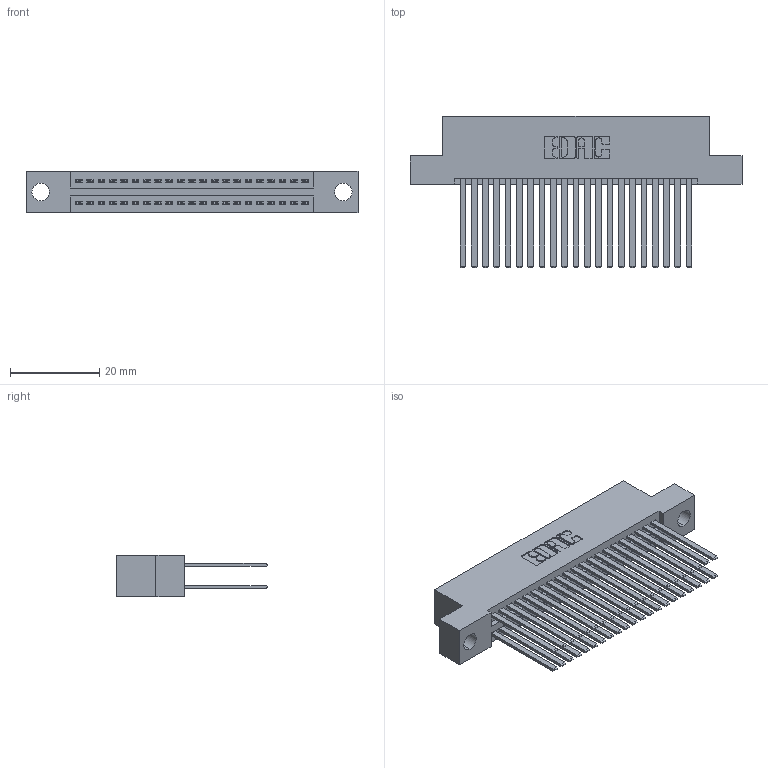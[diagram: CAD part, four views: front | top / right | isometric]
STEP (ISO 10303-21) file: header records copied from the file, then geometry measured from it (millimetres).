
FILE_DESCRIPTION (( 'STEP AP203' ), '1' );
FILE_NAME ('395-042-544-204.STEP', '2018-11-15T11:26:29', ( '' ), ( '' ), 'SwSTEP 2.0', 'SolidWorks 2016', '' );
FILE_SCHEMA (( 'CONFIG_CONTROL_DESIGN' ));
Length unit declared in the file: inch
Products named in the file (3): 345-292-001_345-293-144; 395-042-544-204; 345 Part_Flush Mounting Lugs - 0.156 Dia-TH
Assembly tree (43 placements, depth 2):
  395-042-544-204
    345 Part_Flush Mounting Lugs - 0.156 Dia-TH
    345-292-001_345-293-144  x42
Bounding box: 74.55 x 33.96 x 9.4 mm (x, y, z)
Volume: 7547.7 mm3; surface area: 12290.9 mm2
Topology: 43 solids, 43 shells, 1974 faces, 5843 edges, 3838 vertices
Faces by surface type: plane 1298, cylinder 676
Entity records: 19123 total; most frequent: CARTESIAN_POINT 3224, ORIENTED_EDGE 3158, DIRECTION 2867, EDGE_CURVE 1579, VECTOR 1367, LINE 1367, VERTEX_POINT 1050, AXIS2_PLACEMENT_3D 750
